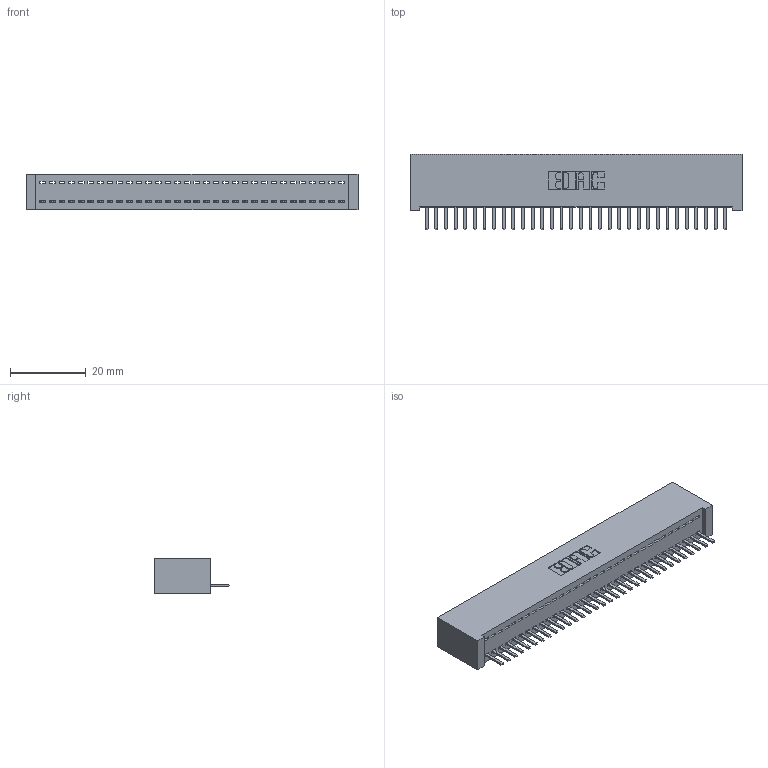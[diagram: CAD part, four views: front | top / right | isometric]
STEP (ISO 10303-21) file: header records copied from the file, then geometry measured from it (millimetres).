
FILE_DESCRIPTION (( 'STEP AP203' ), '1' );
FILE_NAME ('342-032-520-101.STEP', '2019-10-02T06:00:59', ( '' ), ( '' ), 'SwSTEP 2.0', 'SolidWorks 2016', '' );
FILE_SCHEMA (( 'CONFIG_CONTROL_DESIGN' ));
Length unit declared in the file: inch
Products named in the file (3): 345-292-001_345-293-120; 342-032-520-101; 342 Part_Lugless
Assembly tree (33 placements, depth 2):
  342-032-520-101
    342 Part_Lugless
    345-292-001_345-293-120  x32
Bounding box: 87.53 x 20.02 x 9.4 mm (x, y, z)
Volume: 7954.6 mm3; surface area: 11523.1 mm2
Topology: 33 solids, 33 shells, 2086 faces, 6163 edges, 4022 vertices
Faces by surface type: plane 1470, cylinder 616
Entity records: 20561 total; most frequent: CARTESIAN_POINT 3566, ORIENTED_EDGE 3522, DIRECTION 3009, EDGE_CURVE 1761, LINE 1637, VECTOR 1637, VERTEX_POINT 1170, AXIS2_PLACEMENT_3D 686
